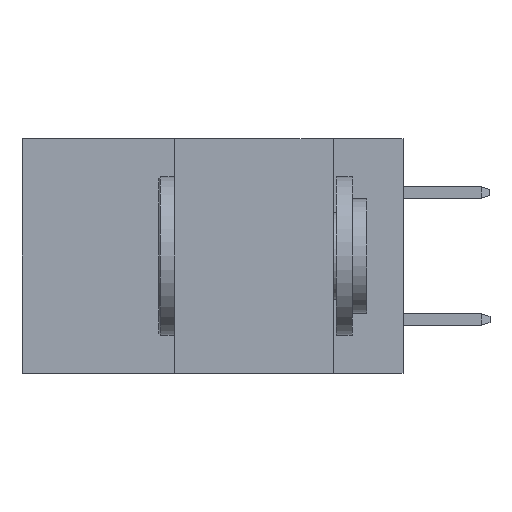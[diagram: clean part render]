
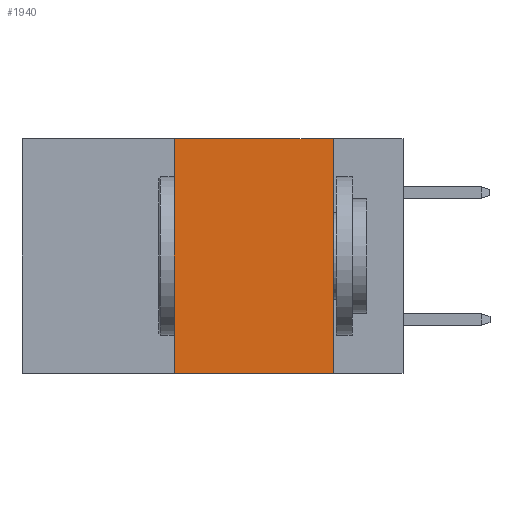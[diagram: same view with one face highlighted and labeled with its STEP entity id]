
A CAD part, left-side view. The second image highlights one B-rep face of the part: STEP entity #1940.
In plain terms, the highlighted planar face has unit normal (-1, 0, 0).
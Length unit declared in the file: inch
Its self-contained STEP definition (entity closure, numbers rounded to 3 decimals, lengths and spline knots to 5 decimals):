
#142 = AXIS2_PLACEMENT_3D ( 'NONE', #6078, #1861, #1646 ) ;
#1149 = EDGE_LOOP ( 'NONE', ( #3422, #8205, #9804, #2114 ) ) ;
#1646 = DIRECTION ( 'NONE',  ( 0., 0., -1. ) ) ;
#1647 = VECTOR ( 'NONE', #3500, 39.37008 ) ;
#1861 = DIRECTION ( 'NONE',  ( 1., 0., 0. ) ) ;
#1940 = ADVANCED_FACE ( 'NONE', ( #9575 ), #10196, .F. ) ;
#2114 = ORIENTED_EDGE ( 'NONE', *, *, #3222, .T. ) ;
#2581 = EDGE_CURVE ( 'NONE', #9020, #4272, #7868, .T. ) ;
#3110 = CARTESIAN_POINT ( 'NONE',  ( 0., 0.11, -0.37 ) ) ;
#3161 = CARTESIAN_POINT ( 'NONE',  ( 0., 0.36, -0.37 ) ) ;
#3222 = EDGE_CURVE ( 'NONE', #3621, #4272, #4979, .T. ) ;
#3422 = ORIENTED_EDGE ( 'NONE', *, *, #2581, .F. ) ;
#3500 = DIRECTION ( 'NONE',  ( 0., -1., 0. ) ) ;
#3576 = CARTESIAN_POINT ( 'NONE',  ( 0., 0.36, 0. ) ) ;
#3621 = VERTEX_POINT ( 'NONE', #3161 ) ;
#3698 = DIRECTION ( 'NONE',  ( 0., 0., -1. ) ) ;
#3868 = EDGE_CURVE ( 'NONE', #9064, #9020, #5247, .T. ) ;
#4272 = VERTEX_POINT ( 'NONE', #3110 ) ;
#4403 = CARTESIAN_POINT ( 'NONE',  ( 0., 0.6, 0. ) ) ;
#4656 = CARTESIAN_POINT ( 'NONE',  ( 0., 0.11, 0. ) ) ;
#4979 = LINE ( 'NONE', #9435, #5399 ) ;
#5247 = LINE ( 'NONE', #4403, #1647 ) ;
#5399 = VECTOR ( 'NONE', #6894, 39.37008 ) ;
#5735 = EDGE_CURVE ( 'NONE', #3621, #9064, #7120, .T. ) ;
#6078 = CARTESIAN_POINT ( 'NONE',  ( 0., 0.6, 0. ) ) ;
#6224 = DIRECTION ( 'NONE',  ( 0., 0., 1. ) ) ;
#6225 = VECTOR ( 'NONE', #3698, 39.37008 ) ;
#6894 = DIRECTION ( 'NONE',  ( 0., -1., 0. ) ) ;
#7006 = VECTOR ( 'NONE', #6224, 39.37008 ) ;
#7120 = LINE ( 'NONE', #3576, #7006 ) ;
#7868 = LINE ( 'NONE', #4656, #6225 ) ;
#8205 = ORIENTED_EDGE ( 'NONE', *, *, #3868, .F. ) ;
#8639 = CARTESIAN_POINT ( 'NONE',  ( 0., 0.11, 0. ) ) ;
#9020 = VERTEX_POINT ( 'NONE', #8639 ) ;
#9064 = VERTEX_POINT ( 'NONE', #9538 ) ;
#9435 = CARTESIAN_POINT ( 'NONE',  ( 0., 0.6, -0.37 ) ) ;
#9538 = CARTESIAN_POINT ( 'NONE',  ( 0., 0.36, 0. ) ) ;
#9575 = FACE_OUTER_BOUND ( 'NONE', #1149, .T. ) ;
#9804 = ORIENTED_EDGE ( 'NONE', *, *, #5735, .F. ) ;
#10196 = PLANE ( 'NONE',  #142 ) ;
